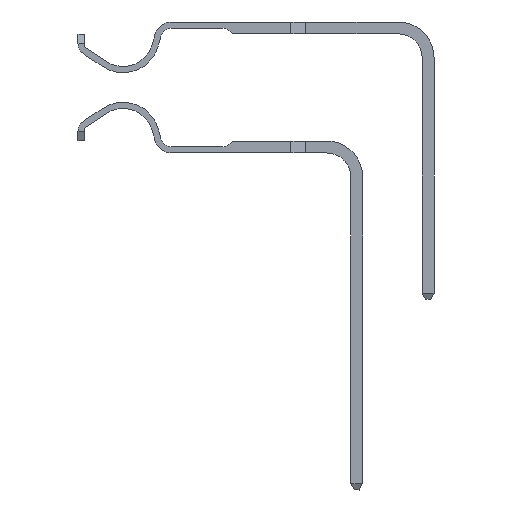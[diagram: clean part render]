
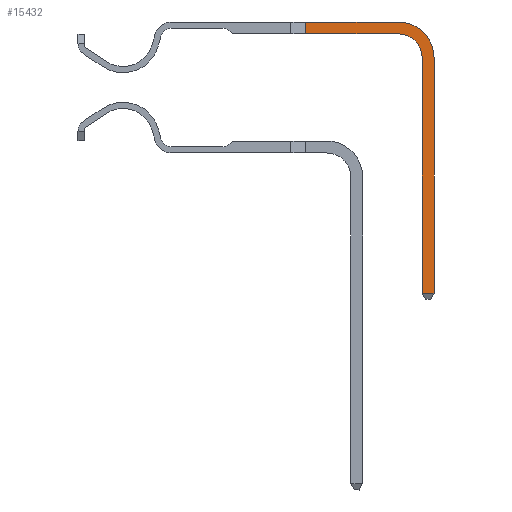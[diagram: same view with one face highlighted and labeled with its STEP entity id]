
A CAD part, left-side view. The second image highlights one B-rep face of the part: STEP entity #15432.
In plain terms, the highlighted face is planar.
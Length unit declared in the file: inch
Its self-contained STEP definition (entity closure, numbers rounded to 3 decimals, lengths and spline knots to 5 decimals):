
#115 = CARTESIAN_POINT ( 'NONE',  ( 0.61115, 0.0875, -0.0125 ) ) ;
#142 = CARTESIAN_POINT ( 'NONE',  ( 0.80571, 0.0375, -0.0125 ) ) ;
#599 = EDGE_CURVE ( 'NONE', #1022, #4721, #8610, .T. ) ;
#803 = ORIENTED_EDGE ( 'NONE', *, *, #22169, .T. ) ;
#1002 = AXIS2_PLACEMENT_3D ( 'NONE', #23867, #11755, #25868 ) ;
#1022 = VERTEX_POINT ( 'NONE', #142 ) ;
#1518 = EDGE_CURVE ( 'NONE', #11944, #18958, #24713, .T. ) ;
#1565 = VERTEX_POINT ( 'NONE', #14629 ) ;
#1610 = DIRECTION ( 'NONE',  ( 0., -1., 0. ) ) ;
#2218 = EDGE_CURVE ( 'NONE', #21990, #11944, #16455, .T. ) ;
#2517 = ORIENTED_EDGE ( 'NONE', *, *, #599, .T. ) ;
#3635 = EDGE_CURVE ( 'NONE', #4721, #1565, #18575, .T. ) ;
#4137 = ORIENTED_EDGE ( 'NONE', *, *, #8491, .T. ) ;
#4593 = DIRECTION ( 'NONE',  ( -1., 0., 0. ) ) ;
#4721 = VERTEX_POINT ( 'NONE', #15875 ) ;
#5697 = LINE ( 'NONE', #20184, #25325 ) ;
#6206 = CARTESIAN_POINT ( 'NONE',  ( 0.80571, 0.582, -0.0125 ) ) ;
#6987 = CARTESIAN_POINT ( 'NONE',  ( 0.58021, 0.0125, -0.0125 ) ) ;
#7709 = EDGE_LOOP ( 'NONE', ( #20591, #803, #23134, #12360, #13613, #8200, #4137, #2517 ) ) ;
#8016 = DIRECTION ( 'NONE',  ( 1., 0., 0. ) ) ;
#8200 = ORIENTED_EDGE ( 'NONE', *, *, #1518, .T. ) ;
#8491 = EDGE_CURVE ( 'NONE', #18958, #1022, #5697, .T. ) ;
#8530 = VECTOR ( 'NONE', #14218, 39.37008 ) ;
#8610 = CIRCLE ( 'NONE', #11770, 0.05 ) ;
#9021 = DIRECTION ( 'NONE',  ( 1., 0., 0. ) ) ;
#9405 = DIRECTION ( 'NONE',  ( 0., 0., 1. ) ) ;
#10009 = CARTESIAN_POINT ( 'NONE',  ( 0.80571, 0.0875, -0.0125 ) ) ;
#10541 = VERTEX_POINT ( 'NONE', #11968 ) ;
#11755 = DIRECTION ( 'NONE',  ( 0., 0., -1. ) ) ;
#11770 = AXIS2_PLACEMENT_3D ( 'NONE', #10009, #22378, #9021 ) ;
#11944 = VERTEX_POINT ( 'NONE', #17980 ) ;
#11968 = CARTESIAN_POINT ( 'NONE',  ( 0.88071, 0.582, -0.0125 ) ) ;
#12360 = ORIENTED_EDGE ( 'NONE', *, *, #23965, .T. ) ;
#13613 = ORIENTED_EDGE ( 'NONE', *, *, #2218, .T. ) ;
#13678 = FACE_OUTER_BOUND ( 'NONE', #7709, .T. ) ;
#14218 = DIRECTION ( 'NONE',  ( 0., 1., 0. ) ) ;
#14629 = CARTESIAN_POINT ( 'NONE',  ( 0.85571, 0.582, -0.0125 ) ) ;
#14769 = CARTESIAN_POINT ( 'NONE',  ( 0.85571, 0.0875, -0.0125 ) ) ;
#15432 = ADVANCED_FACE ( 'NONE', ( #13678 ), #17466, .F. ) ;
#15875 = CARTESIAN_POINT ( 'NONE',  ( 0.85571, 0.0875, -0.0125 ) ) ;
#16455 = LINE ( 'NONE', #6987, #21874 ) ;
#17286 = VECTOR ( 'NONE', #20408, 39.37008 ) ;
#17466 = PLANE ( 'NONE',  #22911 ) ;
#17694 = CARTESIAN_POINT ( 'NONE',  ( 0.88071, 0.0875, -0.0125 ) ) ;
#17962 = VECTOR ( 'NONE', #24866, 39.37008 ) ;
#17980 = CARTESIAN_POINT ( 'NONE',  ( 0.61115, 0.0125, -0.0125 ) ) ;
#18532 = EDGE_CURVE ( 'NONE', #10541, #19223, #23405, .T. ) ;
#18555 = LINE ( 'NONE', #6206, #17286 ) ;
#18575 = LINE ( 'NONE', #14769, #17962 ) ;
#18958 = VERTEX_POINT ( 'NONE', #19717 ) ;
#19223 = VERTEX_POINT ( 'NONE', #17694 ) ;
#19530 = CARTESIAN_POINT ( 'NONE',  ( 0.80571, 0.0125, -0.0125 ) ) ;
#19717 = CARTESIAN_POINT ( 'NONE',  ( 0.61115, 0.0375, -0.0125 ) ) ;
#20184 = CARTESIAN_POINT ( 'NONE',  ( 0.58021, 0.0375, -0.0125 ) ) ;
#20408 = DIRECTION ( 'NONE',  ( 1., 0., 0. ) ) ;
#20591 = ORIENTED_EDGE ( 'NONE', *, *, #3635, .T. ) ;
#21577 = CARTESIAN_POINT ( 'NONE',  ( 0.80571, 0.0875, -0.0125 ) ) ;
#21874 = VECTOR ( 'NONE', #4593, 39.37008 ) ;
#21990 = VERTEX_POINT ( 'NONE', #19530 ) ;
#22146 = VECTOR ( 'NONE', #1610, 39.37008 ) ;
#22169 = EDGE_CURVE ( 'NONE', #1565, #10541, #18555, .T. ) ;
#22296 = CIRCLE ( 'NONE', #1002, 0.075 ) ;
#22378 = DIRECTION ( 'NONE',  ( 0., 0., 1. ) ) ;
#22911 = AXIS2_PLACEMENT_3D ( 'NONE', #21577, #9405, #23591 ) ;
#23134 = ORIENTED_EDGE ( 'NONE', *, *, #18532, .T. ) ;
#23405 = LINE ( 'NONE', #25833, #22146 ) ;
#23591 = DIRECTION ( 'NONE',  ( 1., 0., 0. ) ) ;
#23867 = CARTESIAN_POINT ( 'NONE',  ( 0.80571, 0.0875, -0.0125 ) ) ;
#23965 = EDGE_CURVE ( 'NONE', #19223, #21990, #22296, .T. ) ;
#24713 = LINE ( 'NONE', #115, #8530 ) ;
#24866 = DIRECTION ( 'NONE',  ( 0., 1., 0. ) ) ;
#25325 = VECTOR ( 'NONE', #8016, 39.37008 ) ;
#25833 = CARTESIAN_POINT ( 'NONE',  ( 0.88071, 0.0875, -0.0125 ) ) ;
#25868 = DIRECTION ( 'NONE',  ( 1., 0., 0. ) ) ;
